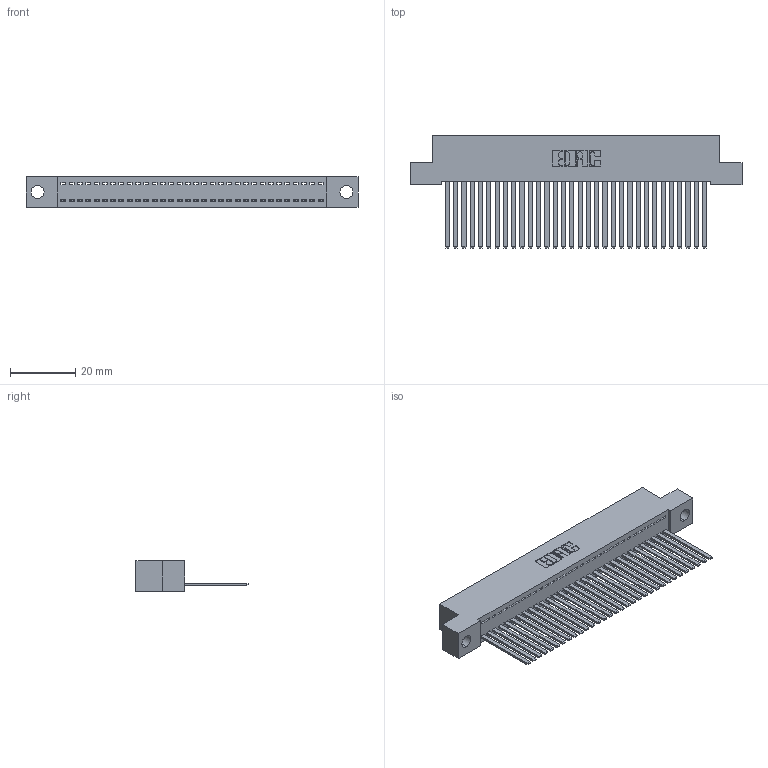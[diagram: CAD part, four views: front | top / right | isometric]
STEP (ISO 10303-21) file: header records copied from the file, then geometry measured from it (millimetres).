
FILE_DESCRIPTION (( 'STEP AP203' ), '1' );
FILE_NAME ('392-032-544-104.STEP', '2018-08-16T00:12:11', ( '' ), ( '' ), 'SwSTEP 2.0', 'SolidWorks 2016', '' );
FILE_SCHEMA (( 'CONFIG_CONTROL_DESIGN' ));
Length unit declared in the file: inch
Products named in the file (3): 342 Part_.156 TH; 345-292-001_345-293-144; 392-032-544-104
Assembly tree (33 placements, depth 2):
  392-032-544-104
    342 Part_.156 TH
    345-292-001_345-293-144  x32
Bounding box: 101.6 x 34.3 x 9.4 mm (x, y, z)
Volume: 9155 mm3; surface area: 14130.6 mm2
Topology: 33 solids, 33 shells, 1774 faces, 5355 edges, 3526 vertices
Faces by surface type: plane 1282, cylinder 492
Entity records: 20543 total; most frequent: CARTESIAN_POINT 3550, ORIENTED_EDGE 3518, DIRECTION 3011, EDGE_CURVE 1759, VECTOR 1635, LINE 1635, VERTEX_POINT 1170, AXIS2_PLACEMENT_3D 688
